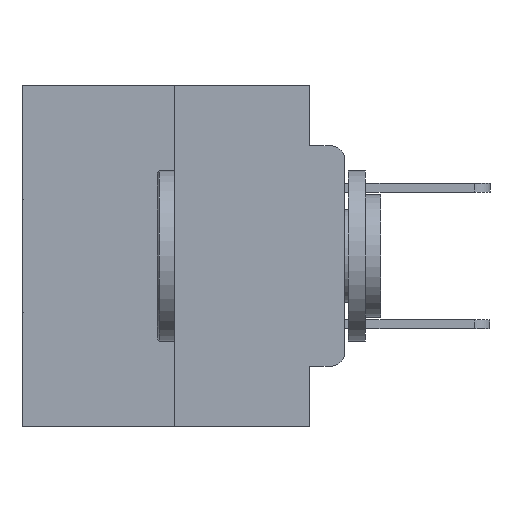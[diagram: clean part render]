
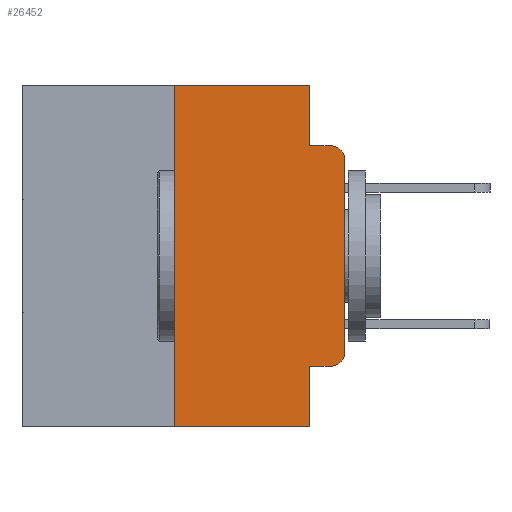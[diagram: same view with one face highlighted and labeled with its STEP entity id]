
A CAD part, left-side view. The second image highlights one B-rep face of the part: STEP entity #26452.
In plain terms, the highlighted planar face has unit normal (-1, 0, 0).
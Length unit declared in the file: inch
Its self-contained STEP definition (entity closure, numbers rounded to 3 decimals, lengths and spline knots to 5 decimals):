
#89 = VERTEX_POINT ( 'NONE', #11478 ) ;
#133 = DIRECTION ( 'NONE',  ( 0., 0., -1. ) ) ;
#136 = AXIS2_PLACEMENT_3D ( 'NONE', #23500, #4229, #19279 ) ;
#270 = VERTEX_POINT ( 'NONE', #14563 ) ;
#508 = VERTEX_POINT ( 'NONE', #18100 ) ;
#561 = EDGE_CURVE ( 'NONE', #5488, #8482, #25478, .T. ) ;
#568 = CARTESIAN_POINT ( 'NONE',  ( 0., 0., -0.3915 ) ) ;
#609 = LINE ( 'NONE', #11637, #22995 ) ;
#1247 = VERTEX_POINT ( 'NONE', #21461 ) ;
#1432 = VECTOR ( 'NONE', #4547, 39.37008 ) ;
#1500 = CARTESIAN_POINT ( 'NONE',  ( 0., 0.473, -0.5 ) ) ;
#1602 = LINE ( 'NONE', #1500, #23935 ) ;
#1681 = CARTESIAN_POINT ( 'NONE',  ( 0., 0.25, -0.5 ) ) ;
#2078 = EDGE_CURVE ( 'NONE', #24772, #89, #13697, .T. ) ;
#2103 = AXIS2_PLACEMENT_3D ( 'NONE', #20016, #7207, #22170 ) ;
#2624 = CARTESIAN_POINT ( 'NONE',  ( 0., 0., 0. ) ) ;
#3063 = CARTESIAN_POINT ( 'NONE',  ( 0., 0.051, -0.5 ) ) ;
#3123 = DIRECTION ( 'NONE',  ( 0., 0., -1. ) ) ;
#3432 = LINE ( 'NONE', #25065, #14232 ) ;
#4113 = VECTOR ( 'NONE', #9047, 39.37008 ) ;
#4229 = DIRECTION ( 'NONE',  ( 1., 0., 0. ) ) ;
#4547 = DIRECTION ( 'NONE',  ( 0., 0., 1. ) ) ;
#4628 = VERTEX_POINT ( 'NONE', #568 ) ;
#5101 = EDGE_CURVE ( 'NONE', #4628, #270, #19364, .T. ) ;
#5283 = CARTESIAN_POINT ( 'NONE',  ( 0., 0.02, -0.1085 ) ) ;
#5488 = VERTEX_POINT ( 'NONE', #25408 ) ;
#6569 = EDGE_CURVE ( 'NONE', #270, #8482, #17969, .T. ) ;
#6804 = ORIENTED_EDGE ( 'NONE', *, *, #5101, .T. ) ;
#7207 = DIRECTION ( 'NONE',  ( -1., 0., 0. ) ) ;
#7346 = VECTOR ( 'NONE', #133, 39.37008 ) ;
#7479 = DIRECTION ( 'NONE',  ( 0., 0., -1. ) ) ;
#7988 = VERTEX_POINT ( 'NONE', #8251 ) ;
#7998 = VECTOR ( 'NONE', #17793, 39.37008 ) ;
#8251 = CARTESIAN_POINT ( 'NONE',  ( 0., 0.051, -0.4115 ) ) ;
#8482 = VERTEX_POINT ( 'NONE', #14177 ) ;
#8881 = EDGE_LOOP ( 'NONE', ( #6804, #20225, #12863, #16502, #23969, #22660, #18687, #9313, #22036, #21751 ) ) ;
#9047 = DIRECTION ( 'NONE',  ( 0., -1., 0. ) ) ;
#9313 = ORIENTED_EDGE ( 'NONE', *, *, #24329, .F. ) ;
#11065 = DIRECTION ( 'NONE',  ( 0., -1., 0. ) ) ;
#11478 = CARTESIAN_POINT ( 'NONE',  ( 0., 0.25, 0. ) ) ;
#11637 = CARTESIAN_POINT ( 'NONE',  ( 0., 0.051, 0. ) ) ;
#11894 = AXIS2_PLACEMENT_3D ( 'NONE', #5283, #20289, #7479 ) ;
#12863 = ORIENTED_EDGE ( 'NONE', *, *, #561, .F. ) ;
#13697 = LINE ( 'NONE', #13778, #1432 ) ;
#13778 = CARTESIAN_POINT ( 'NONE',  ( 0., 0.25, 0. ) ) ;
#14177 = CARTESIAN_POINT ( 'NONE',  ( 0., 0.02, -0.0885 ) ) ;
#14232 = VECTOR ( 'NONE', #27221, 39.37008 ) ;
#14253 = EDGE_CURVE ( 'NONE', #508, #4628, #23338, .T. ) ;
#14563 = CARTESIAN_POINT ( 'NONE',  ( 0., 0., -0.1085 ) ) ;
#14835 = EDGE_CURVE ( 'NONE', #89, #1247, #3432, .T. ) ;
#15548 = EDGE_CURVE ( 'NONE', #24772, #19594, #1602, .T. ) ;
#16502 = ORIENTED_EDGE ( 'NONE', *, *, #25770, .F. ) ;
#17134 = PLANE ( 'NONE',  #136 ) ;
#17303 = FACE_OUTER_BOUND ( 'NONE', #8881, .T. ) ;
#17484 = CARTESIAN_POINT ( 'NONE',  ( 0., 0.051, 0. ) ) ;
#17793 = DIRECTION ( 'NONE',  ( 0., 0., 1. ) ) ;
#17969 = CIRCLE ( 'NONE', #11894, 0.02 ) ;
#18100 = CARTESIAN_POINT ( 'NONE',  ( 0., 0.02, -0.4115 ) ) ;
#18366 = CARTESIAN_POINT ( 'NONE',  ( 0., 0.051, -0.0885 ) ) ;
#18687 = ORIENTED_EDGE ( 'NONE', *, *, #15548, .T. ) ;
#19279 = DIRECTION ( 'NONE',  ( 0., 0., -1. ) ) ;
#19364 = LINE ( 'NONE', #2624, #7998 ) ;
#19594 = VERTEX_POINT ( 'NONE', #3063 ) ;
#19707 = CARTESIAN_POINT ( 'NONE',  ( 0., 0.051, -0.4115 ) ) ;
#20016 = CARTESIAN_POINT ( 'NONE',  ( 0., 0.02, -0.3915 ) ) ;
#20225 = ORIENTED_EDGE ( 'NONE', *, *, #6569, .T. ) ;
#20289 = DIRECTION ( 'NONE',  ( -1., 0., 0. ) ) ;
#21461 = CARTESIAN_POINT ( 'NONE',  ( 0., 0.051, 0. ) ) ;
#21751 = ORIENTED_EDGE ( 'NONE', *, *, #14253, .T. ) ;
#22036 = ORIENTED_EDGE ( 'NONE', *, *, #27200, .T. ) ;
#22170 = DIRECTION ( 'NONE',  ( 0., 0., -1. ) ) ;
#22660 = ORIENTED_EDGE ( 'NONE', *, *, #2078, .F. ) ;
#22995 = VECTOR ( 'NONE', #3123, 39.37008 ) ;
#23152 = DIRECTION ( 'NONE',  ( 0., -1., 0. ) ) ;
#23338 = CIRCLE ( 'NONE', #2103, 0.02 ) ;
#23500 = CARTESIAN_POINT ( 'NONE',  ( 0., 0.473, 0. ) ) ;
#23935 = VECTOR ( 'NONE', #23152, 39.37008 ) ;
#23969 = ORIENTED_EDGE ( 'NONE', *, *, #14835, .F. ) ;
#24329 = EDGE_CURVE ( 'NONE', #7988, #19594, #24416, .T. ) ;
#24416 = LINE ( 'NONE', #17484, #7346 ) ;
#24772 = VERTEX_POINT ( 'NONE', #1681 ) ;
#24808 = VECTOR ( 'NONE', #11065, 39.37008 ) ;
#25065 = CARTESIAN_POINT ( 'NONE',  ( 0., 0.473, 0. ) ) ;
#25408 = CARTESIAN_POINT ( 'NONE',  ( 0., 0.051, -0.0885 ) ) ;
#25478 = LINE ( 'NONE', #18366, #24808 ) ;
#25770 = EDGE_CURVE ( 'NONE', #1247, #5488, #609, .T. ) ;
#26452 = ADVANCED_FACE ( 'NONE', ( #17303 ), #17134, .F. ) ;
#26975 = LINE ( 'NONE', #19707, #4113 ) ;
#27200 = EDGE_CURVE ( 'NONE', #7988, #508, #26975, .T. ) ;
#27221 = DIRECTION ( 'NONE',  ( 0., -1., 0. ) ) ;
